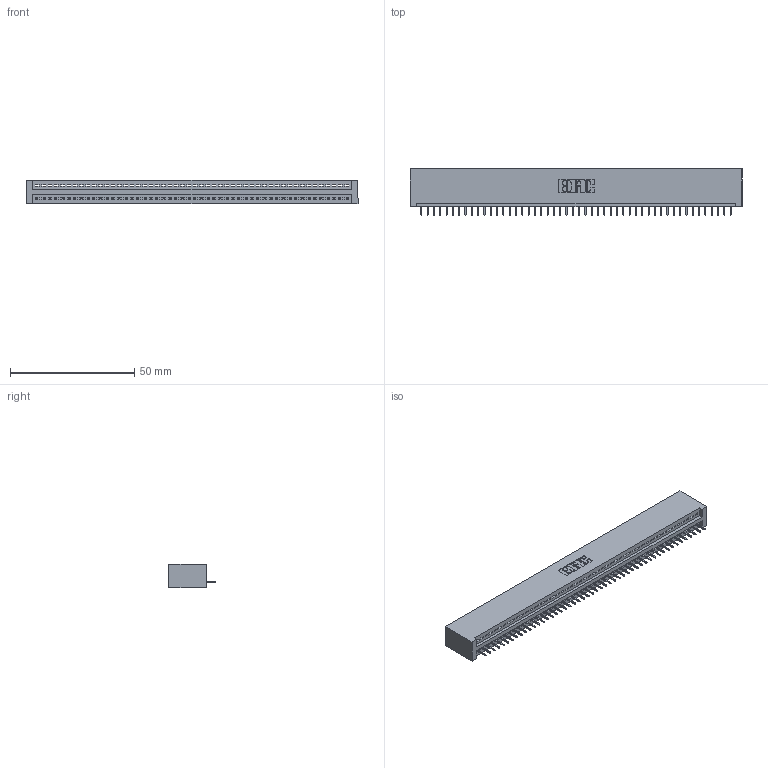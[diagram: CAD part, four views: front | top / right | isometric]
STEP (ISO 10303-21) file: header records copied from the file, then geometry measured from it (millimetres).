
FILE_DESCRIPTION (( 'STEP AP203' ), '1' );
FILE_NAME ('895-050-525-101.STEP', '2020-09-27T09:17:24', ( '' ), ( '' ), 'SwSTEP 2.0', 'SolidWorks 2020', '' );
FILE_SCHEMA (( 'CONFIG_CONTROL_DESIGN' ));
Length unit declared in the file: inch
Products named in the file (3): 845 Part_No Mounting Lugs; 345-292-001_345-293-125; 895-050-525-101
Assembly tree (51 placements, depth 2):
  895-050-525-101
    845 Part_No Mounting Lugs
    345-292-001_345-293-125  x50
Bounding box: 133.6 x 18.72 x 9.4 mm (x, y, z)
Volume: 13135.6 mm3; surface area: 17074.1 mm2
Topology: 51 solids, 51 shells, 3218 faces, 9317 edges, 6010 vertices
Faces by surface type: plane 2376, cylinder 842
Entity records: 36351 total; most frequent: CARTESIAN_POINT 6302, ORIENTED_EDGE 6286, DIRECTION 5487, EDGE_CURVE 3143, LINE 2823, VECTOR 2823, VERTEX_POINT 2090, AXIS2_PLACEMENT_3D 1332
